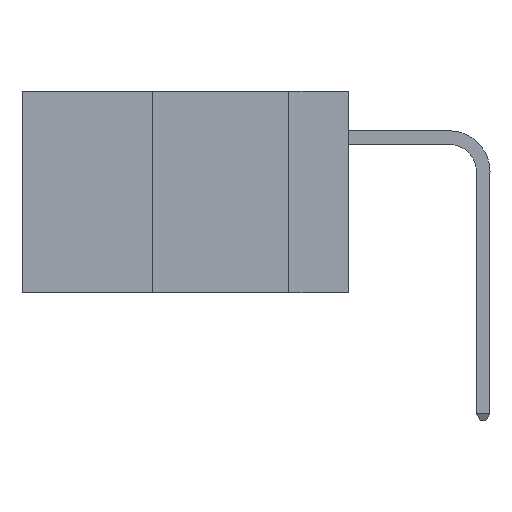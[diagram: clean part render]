
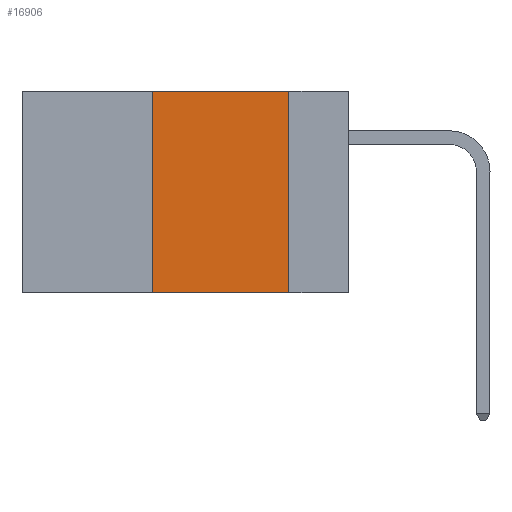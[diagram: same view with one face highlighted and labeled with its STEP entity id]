
A CAD part, left-side view. The second image highlights one B-rep face of the part: STEP entity #16906.
In plain terms, the highlighted planar face has unit normal (-1, 0, 0).
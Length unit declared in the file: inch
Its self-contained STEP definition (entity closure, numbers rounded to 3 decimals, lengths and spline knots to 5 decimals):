
#78 = PLANE ( 'NONE',  #12540 ) ;
#942 = EDGE_CURVE ( 'NONE', #12858, #15840, #12087, .T. ) ;
#1636 = EDGE_CURVE ( 'NONE', #20520, #10459, #11773, .T. ) ;
#1794 = CARTESIAN_POINT ( 'NONE',  ( 0., 0.36, 0. ) ) ;
#1896 = DIRECTION ( 'NONE',  ( 0., 0., -1. ) ) ;
#2220 = DIRECTION ( 'NONE',  ( 0., -1., 0. ) ) ;
#2478 = VECTOR ( 'NONE', #2220, 39.37008 ) ;
#3053 = ORIENTED_EDGE ( 'NONE', *, *, #20960, .F. ) ;
#3077 = ORIENTED_EDGE ( 'NONE', *, *, #942, .F. ) ;
#3169 = ORIENTED_EDGE ( 'NONE', *, *, #5954, .F. ) ;
#3407 = ORIENTED_EDGE ( 'NONE', *, *, #1636, .T. ) ;
#5701 = VECTOR ( 'NONE', #19491, 39.37008 ) ;
#5734 = CARTESIAN_POINT ( 'NONE',  ( 0., 0.6, -0.37 ) ) ;
#5807 = CARTESIAN_POINT ( 'NONE',  ( 0., 0.11, 0. ) ) ;
#5954 = EDGE_CURVE ( 'NONE', #20520, #12858, #6231, .T. ) ;
#6231 = LINE ( 'NONE', #16046, #5701 ) ;
#6835 = VECTOR ( 'NONE', #7614, 39.37008 ) ;
#7475 = VECTOR ( 'NONE', #17451, 39.37008 ) ;
#7614 = DIRECTION ( 'NONE',  ( 0., 0., -1. ) ) ;
#10459 = VERTEX_POINT ( 'NONE', #11929 ) ;
#10909 = LINE ( 'NONE', #17946, #6835 ) ;
#11773 = LINE ( 'NONE', #5734, #2478 ) ;
#11929 = CARTESIAN_POINT ( 'NONE',  ( 0., 0.11, -0.37 ) ) ;
#12087 = LINE ( 'NONE', #12267, #7475 ) ;
#12267 = CARTESIAN_POINT ( 'NONE',  ( 0., 0.6, 0. ) ) ;
#12378 = DIRECTION ( 'NONE',  ( 1., 0., 0. ) ) ;
#12540 = AXIS2_PLACEMENT_3D ( 'NONE', #14031, #12378, #1896 ) ;
#12858 = VERTEX_POINT ( 'NONE', #1794 ) ;
#13728 = CARTESIAN_POINT ( 'NONE',  ( 0., 0.36, -0.37 ) ) ;
#14031 = CARTESIAN_POINT ( 'NONE',  ( 0., 0.6, 0. ) ) ;
#15840 = VERTEX_POINT ( 'NONE', #5807 ) ;
#16046 = CARTESIAN_POINT ( 'NONE',  ( 0., 0.36, 0. ) ) ;
#16906 = ADVANCED_FACE ( 'NONE', ( #17269 ), #78, .F. ) ;
#17269 = FACE_OUTER_BOUND ( 'NONE', #19508, .T. ) ;
#17451 = DIRECTION ( 'NONE',  ( 0., -1., 0. ) ) ;
#17946 = CARTESIAN_POINT ( 'NONE',  ( 0., 0.11, 0. ) ) ;
#19491 = DIRECTION ( 'NONE',  ( 0., 0., 1. ) ) ;
#19508 = EDGE_LOOP ( 'NONE', ( #3053, #3077, #3169, #3407 ) ) ;
#20520 = VERTEX_POINT ( 'NONE', #13728 ) ;
#20960 = EDGE_CURVE ( 'NONE', #15840, #10459, #10909, .T. ) ;
